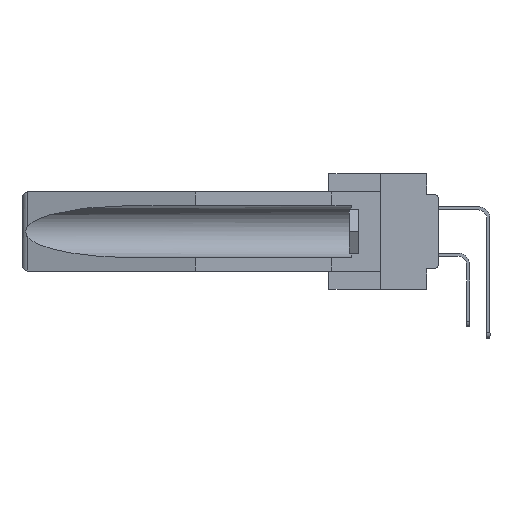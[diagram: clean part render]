
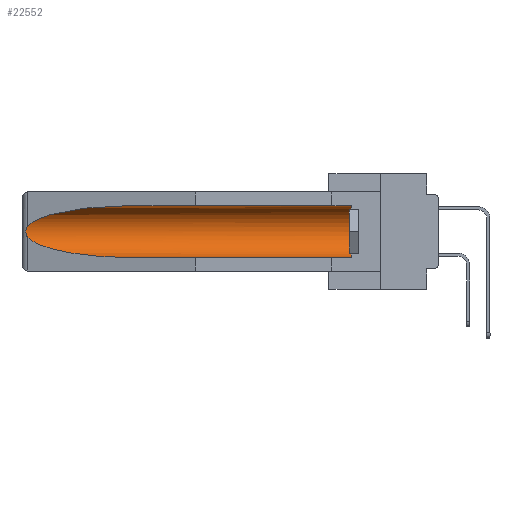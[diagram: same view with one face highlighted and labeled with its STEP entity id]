
A CAD part, left-side view. The second image highlights one B-rep face of the part: STEP entity #22552.
In plain terms, the highlighted cylindrical face has radius 2.857 mm (diameter 5.715 mm), a partial arc.
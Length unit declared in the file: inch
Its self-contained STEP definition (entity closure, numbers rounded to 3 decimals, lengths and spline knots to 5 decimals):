
#965 = CARTESIAN_POINT ( 'NONE',  ( 0.26537, 1.52718, -0.19328 ) ) ;
#1713 = VERTEX_POINT ( 'NONE', #28807 ) ;
#2048 = VERTEX_POINT ( 'NONE', #3319 ) ;
#3319 = CARTESIAN_POINT ( 'NONE',  ( 0.155, 0.126, -0.284 ) ) ;
#4020 = ORIENTED_EDGE ( 'NONE', *, *, #12848, .T. ) ;
#4957 = CARTESIAN_POINT ( 'NONE',  ( 0.155, -0.30754, -0.284 ) ) ;
#5764 = ORIENTED_EDGE ( 'NONE', *, *, #22103, .T. ) ;
#6625 = CARTESIAN_POINT ( 'NONE',  ( 0.25451, 1.48313, -0.09465 ) ) ;
#6918 = FACE_OUTER_BOUND ( 'NONE', #17841, .T. ) ;
#7128 = CIRCLE ( 'NONE', #20573, 0.1125 ) ;
#7723 = CARTESIAN_POINT ( 'NONE',  ( 0.26655, 1.53094, -0.18657 ) ) ;
#8485 = ORIENTED_EDGE ( 'NONE', *, *, #19199, .T. ) ;
#9007 = CARTESIAN_POINT ( 'NONE',  ( 0.155, -0.30754, -0.059 ) ) ;
#10157 = CARTESIAN_POINT ( 'NONE',  ( 0.26537, 1.52718, -0.14972 ) ) ;
#10582 = CARTESIAN_POINT ( 'NONE',  ( 0.21114, 1.30732, -0.284 ) ) ;
#11966 = CYLINDRICAL_SURFACE ( 'NONE', #25050, 0.1125 ) ;
#12132 = CARTESIAN_POINT ( 'NONE',  ( 0.155, 0.126, -0.059 ) ) ;
#12350 = VECTOR ( 'NONE', #20220, 39.37008 ) ;
#12390 =( BOUNDED_CURVE ( )  B_SPLINE_CURVE ( 3, ( #31921, #24484, #6625, #29486 ),
 .UNSPECIFIED., .F., .F. ) 
 B_SPLINE_CURVE_WITH_KNOTS ( ( 4, 4 ),
 ( 4.71239, 6.08839 ),
 .UNSPECIFIED. ) 
 CURVE ( )  GEOMETRIC_REPRESENTATION_ITEM ( )  RATIONAL_B_SPLINE_CURVE ( ( 1., 0.848, 0.848, 1. ) ) 
 REPRESENTATION_ITEM ( '' )  );
#12570 = DIRECTION ( 'NONE',  ( 0., 0., 1. ) ) ;
#12621 = LINE ( 'NONE', #4957, #12350 ) ;
#12769 = CARTESIAN_POINT ( 'NONE',  ( 0.2673, 1.53269, -0.17917 ) ) ;
#12848 = EDGE_CURVE ( 'NONE', #1713, #15502, #28761, .T. ) ;
#14107 = CARTESIAN_POINT ( 'NONE',  ( 0.155, 1.07973, -0.284 ) ) ;
#14327 = VERTEX_POINT ( 'NONE', #14107 ) ;
#14615 = ORIENTED_EDGE ( 'NONE', *, *, #29473, .F. ) ;
#15117 = VECTOR ( 'NONE', #21638, 39.37008 ) ;
#15502 = VERTEX_POINT ( 'NONE', #23503 ) ;
#17841 = EDGE_LOOP ( 'NONE', ( #5764, #4020, #8485, #14615, #21197, #26287 ) ) ;
#18225 = CARTESIAN_POINT ( 'NONE',  ( 0.25451, 1.48313, -0.24835 ) ) ;
#19199 = EDGE_CURVE ( 'NONE', #15502, #14327, #21262, .T. ) ;
#19267 = DIRECTION ( 'NONE',  ( 0., 0., 1. ) ) ;
#19893 = VERTEX_POINT ( 'NONE', #12132 ) ;
#19903 = CARTESIAN_POINT ( 'NONE',  ( 0.2673, 1.5327, -0.16383 ) ) ;
#20053 = CARTESIAN_POINT ( 'NONE',  ( 0.2675, 1.53308, -0.17534 ) ) ;
#20217 = CARTESIAN_POINT ( 'NONE',  ( 0.26597, 1.5296, -0.19026 ) ) ;
#20220 = DIRECTION ( 'NONE',  ( 0., 1., 0. ) ) ;
#20455 = EDGE_CURVE ( 'NONE', #19893, #26332, #24070, .T. ) ;
#20457 = CARTESIAN_POINT ( 'NONE',  ( 0.155, 1.07973, -0.284 ) ) ;
#20573 = AXIS2_PLACEMENT_3D ( 'NONE', #22435, #26811, #12570 ) ;
#21197 = ORIENTED_EDGE ( 'NONE', *, *, #26889, .T. ) ;
#21262 =( BOUNDED_CURVE ( )  B_SPLINE_CURVE ( 3, ( #965, #18225, #10582, #20457 ),
 .UNSPECIFIED., .F., .F. ) 
 B_SPLINE_CURVE_WITH_KNOTS ( ( 4, 4 ),
 ( 0.1948, 1.5708 ),
 .UNSPECIFIED. ) 
 CURVE ( )  GEOMETRIC_REPRESENTATION_ITEM ( )  RATIONAL_B_SPLINE_CURVE ( ( 1., 0.848, 0.848, 1. ) ) 
 REPRESENTATION_ITEM ( '' )  );
#21638 = DIRECTION ( 'NONE',  ( 0., 1., 0. ) ) ;
#21667 = DIRECTION ( 'NONE',  ( 0., 1., 0. ) ) ;
#22103 = EDGE_CURVE ( 'NONE', #26332, #1713, #12390, .T. ) ;
#22321 = CARTESIAN_POINT ( 'NONE',  ( 0.2675, 1.53308, -0.16763 ) ) ;
#22435 = CARTESIAN_POINT ( 'NONE',  ( 0.155, 0.126, -0.1715 ) ) ;
#22552 = ADVANCED_FACE ( 'NONE', ( #6918 ), #11966, .F. ) ;
#23503 = CARTESIAN_POINT ( 'NONE',  ( 0.26537, 1.52718, -0.19328 ) ) ;
#24070 = LINE ( 'NONE', #9007, #15117 ) ;
#24096 = CARTESIAN_POINT ( 'NONE',  ( 0.155, -0.30754, -0.1715 ) ) ;
#24248 = CARTESIAN_POINT ( 'NONE',  ( 0.155, 1.07973, -0.059 ) ) ;
#24484 = CARTESIAN_POINT ( 'NONE',  ( 0.21114, 1.30732, -0.059 ) ) ;
#24924 = CARTESIAN_POINT ( 'NONE',  ( 0.26654, 1.53092, -0.15636 ) ) ;
#25050 = AXIS2_PLACEMENT_3D ( 'NONE', #24096, #21667, #19267 ) ;
#26287 = ORIENTED_EDGE ( 'NONE', *, *, #20455, .T. ) ;
#26332 = VERTEX_POINT ( 'NONE', #24248 ) ;
#26811 = DIRECTION ( 'NONE',  ( 0., -1., 0. ) ) ;
#26889 = EDGE_CURVE ( 'NONE', #2048, #19893, #7128, .T. ) ;
#27334 = CARTESIAN_POINT ( 'NONE',  ( 0.26597, 1.52961, -0.15275 ) ) ;
#27652 = CARTESIAN_POINT ( 'NONE',  ( 0.26537, 1.52718, -0.19328 ) ) ;
#28761 = B_SPLINE_CURVE_WITH_KNOTS ( 'NONE', 3,
 ( #10157, #27334, #24924, #19903, #22321, #20053, #12769, #7723, #20217, #27652 ),
 .UNSPECIFIED., .F., .F.,
 ( 4, 2, 2, 2, 4 ),
 ( 0., 0.00029, 0.00058, 0.00087, 0.00117 ),
 .UNSPECIFIED. ) ;
#28807 = CARTESIAN_POINT ( 'NONE',  ( 0.26537, 1.52718, -0.14972 ) ) ;
#29473 = EDGE_CURVE ( 'NONE', #2048, #14327, #12621, .T. ) ;
#29486 = CARTESIAN_POINT ( 'NONE',  ( 0.26537, 1.52718, -0.14972 ) ) ;
#31921 = CARTESIAN_POINT ( 'NONE',  ( 0.155, 1.07973, -0.059 ) ) ;
